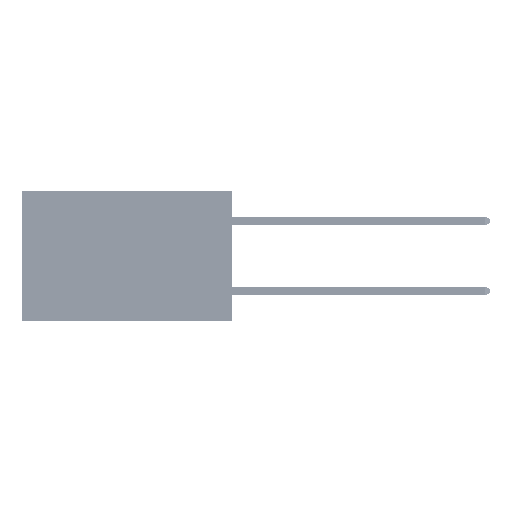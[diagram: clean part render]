
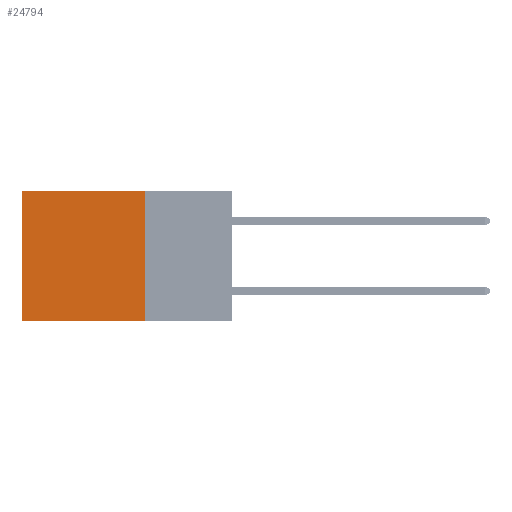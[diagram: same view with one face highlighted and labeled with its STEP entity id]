
A CAD part, left-side view. The second image highlights one B-rep face of the part: STEP entity #24794.
In plain terms, the highlighted planar face has unit normal (-1, 0, 0).
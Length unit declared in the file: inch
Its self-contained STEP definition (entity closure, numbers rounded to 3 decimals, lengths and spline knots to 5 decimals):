
#578 = LINE ( 'NONE', #45012, #39019 ) ;
#1036 = VECTOR ( 'NONE', #49324, 39.37008 ) ;
#2303 = LINE ( 'NONE', #16450, #41964 ) ;
#2366 = ORIENTED_EDGE ( 'NONE', *, *, #46610, .F. ) ;
#3583 = ORIENTED_EDGE ( 'NONE', *, *, #45492, .T. ) ;
#3885 = CARTESIAN_POINT ( 'NONE',  ( 0.2875, 0.6, 0. ) ) ;
#5677 = DIRECTION ( 'NONE',  ( 1., 0., 0. ) ) ;
#5839 = DIRECTION ( 'NONE',  ( 0., 0., -1. ) ) ;
#6446 = LINE ( 'NONE', #14797, #1036 ) ;
#7745 = DIRECTION ( 'NONE',  ( 0., 1., 0. ) ) ;
#11141 = LINE ( 'NONE', #43066, #48341 ) ;
#14797 = CARTESIAN_POINT ( 'NONE',  ( 0.2875, 0.25, 0. ) ) ;
#16286 = DIRECTION ( 'NONE',  ( 0., 0., -1. ) ) ;
#16298 = ORIENTED_EDGE ( 'NONE', *, *, #24371, .T. ) ;
#16450 = CARTESIAN_POINT ( 'NONE',  ( 0.2875, 0.25, 0. ) ) ;
#19690 = EDGE_CURVE ( 'NONE', #35504, #31145, #2303, .T. ) ;
#20765 = FACE_OUTER_BOUND ( 'NONE', #32312, .T. ) ;
#21919 = ORIENTED_EDGE ( 'NONE', *, *, #19690, .F. ) ;
#23448 = AXIS2_PLACEMENT_3D ( 'NONE', #25585, #5677, #5839 ) ;
#24371 = EDGE_CURVE ( 'NONE', #35504, #31704, #6446, .T. ) ;
#24794 = ADVANCED_FACE ( 'NONE', ( #20765 ), #48293, .F. ) ;
#25585 = CARTESIAN_POINT ( 'NONE',  ( 0.2875, 0.25, 0. ) ) ;
#26405 = VERTEX_POINT ( 'NONE', #36977 ) ;
#31145 = VERTEX_POINT ( 'NONE', #35451 ) ;
#31607 = DIRECTION ( 'NONE',  ( 0., 0., -1. ) ) ;
#31704 = VERTEX_POINT ( 'NONE', #3885 ) ;
#32312 = EDGE_LOOP ( 'NONE', ( #3583, #2366, #21919, #16298 ) ) ;
#35451 = CARTESIAN_POINT ( 'NONE',  ( 0.2875, 0.25, -0.37 ) ) ;
#35504 = VERTEX_POINT ( 'NONE', #45957 ) ;
#36977 = CARTESIAN_POINT ( 'NONE',  ( 0.2875, 0.6, -0.37 ) ) ;
#39019 = VECTOR ( 'NONE', #7745, 39.37008 ) ;
#41964 = VECTOR ( 'NONE', #16286, 39.37008 ) ;
#43066 = CARTESIAN_POINT ( 'NONE',  ( 0.2875, 0.6, 0. ) ) ;
#45012 = CARTESIAN_POINT ( 'NONE',  ( 0.2875, 0.25, -0.37 ) ) ;
#45492 = EDGE_CURVE ( 'NONE', #31704, #26405, #11141, .T. ) ;
#45957 = CARTESIAN_POINT ( 'NONE',  ( 0.2875, 0.25, 0. ) ) ;
#46610 = EDGE_CURVE ( 'NONE', #31145, #26405, #578, .T. ) ;
#48293 = PLANE ( 'NONE',  #23448 ) ;
#48341 = VECTOR ( 'NONE', #31607, 39.37008 ) ;
#49324 = DIRECTION ( 'NONE',  ( 0., 1., 0. ) ) ;
